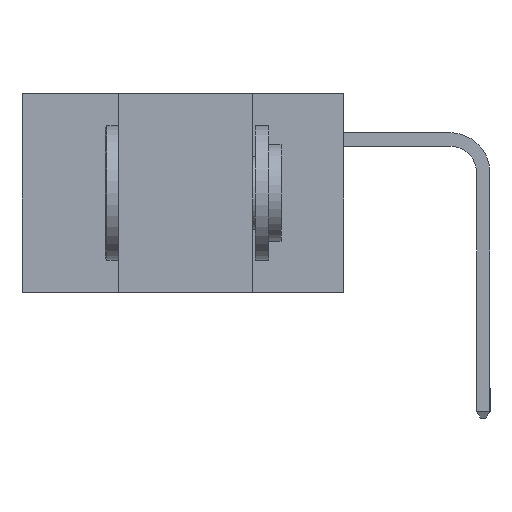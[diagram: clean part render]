
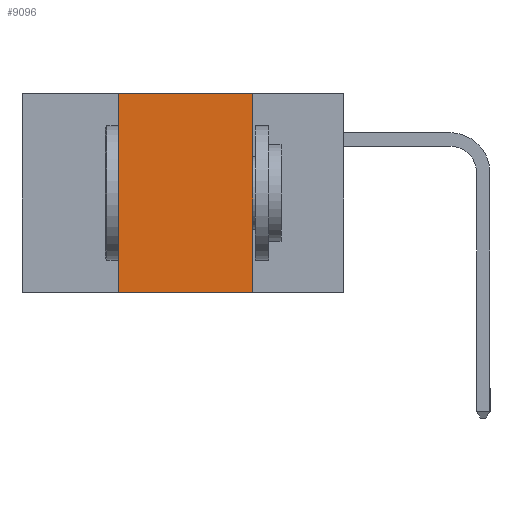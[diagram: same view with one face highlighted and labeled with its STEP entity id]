
A CAD part, left-side view. The second image highlights one B-rep face of the part: STEP entity #9096.
In plain terms, the highlighted planar face has unit normal (-1, 0, 0).
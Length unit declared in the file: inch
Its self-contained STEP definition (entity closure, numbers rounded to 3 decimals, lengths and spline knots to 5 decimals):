
#66 = ORIENTED_EDGE ( 'NONE', *, *, #15750, .T. ) ;
#246 = DIRECTION ( 'NONE',  ( 0., 0., 1. ) ) ;
#342 = VERTEX_POINT ( 'NONE', #3641 ) ;
#683 = FACE_OUTER_BOUND ( 'NONE', #12030, .T. ) ;
#3548 = AXIS2_PLACEMENT_3D ( 'NONE', #12238, #13566, #5558 ) ;
#3641 = CARTESIAN_POINT ( 'NONE',  ( 0., 0.42, -0.37 ) ) ;
#4228 = CARTESIAN_POINT ( 'NONE',  ( 0., 0.42, 0. ) ) ;
#5048 = CARTESIAN_POINT ( 'NONE',  ( 0., 0.6, -0.37 ) ) ;
#5402 = CARTESIAN_POINT ( 'NONE',  ( 0., 0.17, 0. ) ) ;
#5558 = DIRECTION ( 'NONE',  ( 0., 0., -1. ) ) ;
#5593 = VERTEX_POINT ( 'NONE', #12150 ) ;
#5805 = ORIENTED_EDGE ( 'NONE', *, *, #14877, .F. ) ;
#5810 = VERTEX_POINT ( 'NONE', #13839 ) ;
#6169 = CARTESIAN_POINT ( 'NONE',  ( 0., 0.6, 0. ) ) ;
#6217 = VECTOR ( 'NONE', #8876, 39.37008 ) ;
#6391 = DIRECTION ( 'NONE',  ( 0., -1., 0. ) ) ;
#7317 = LINE ( 'NONE', #4228, #14007 ) ;
#8876 = DIRECTION ( 'NONE',  ( 0., -1., 0. ) ) ;
#9096 = ADVANCED_FACE ( 'NONE', ( #683 ), #10893, .F. ) ;
#9386 = ORIENTED_EDGE ( 'NONE', *, *, #13102, .F. ) ;
#9498 = EDGE_CURVE ( 'NONE', #5593, #12948, #14155, .T. ) ;
#9762 = LINE ( 'NONE', #6169, #6217 ) ;
#9978 = VECTOR ( 'NONE', #6391, 39.37008 ) ;
#10599 = ORIENTED_EDGE ( 'NONE', *, *, #9498, .F. ) ;
#10893 = PLANE ( 'NONE',  #3548 ) ;
#11011 = VECTOR ( 'NONE', #14761, 39.37008 ) ;
#12030 = EDGE_LOOP ( 'NONE', ( #10599, #9386, #5805, #66 ) ) ;
#12150 = CARTESIAN_POINT ( 'NONE',  ( 0., 0.17, 0. ) ) ;
#12238 = CARTESIAN_POINT ( 'NONE',  ( 0., 0.6, 0. ) ) ;
#12948 = VERTEX_POINT ( 'NONE', #15242 ) ;
#13102 = EDGE_CURVE ( 'NONE', #5810, #5593, #9762, .T. ) ;
#13566 = DIRECTION ( 'NONE',  ( 1., 0., 0. ) ) ;
#13839 = CARTESIAN_POINT ( 'NONE',  ( 0., 0.42, 0. ) ) ;
#13967 = LINE ( 'NONE', #5048, #9978 ) ;
#14007 = VECTOR ( 'NONE', #246, 39.37008 ) ;
#14155 = LINE ( 'NONE', #5402, #11011 ) ;
#14761 = DIRECTION ( 'NONE',  ( 0., 0., -1. ) ) ;
#14877 = EDGE_CURVE ( 'NONE', #342, #5810, #7317, .T. ) ;
#15242 = CARTESIAN_POINT ( 'NONE',  ( 0., 0.17, -0.37 ) ) ;
#15750 = EDGE_CURVE ( 'NONE', #342, #12948, #13967, .T. ) ;
